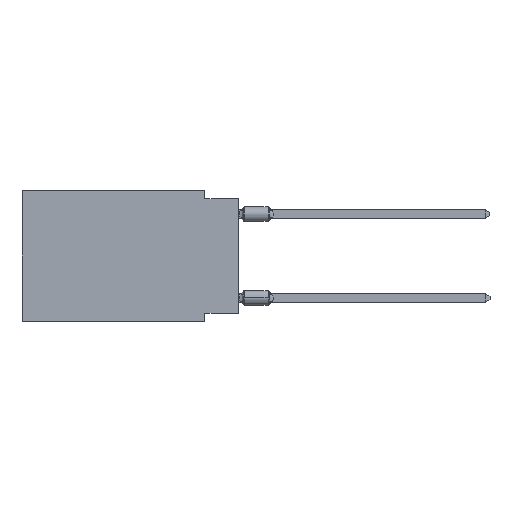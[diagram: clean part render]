
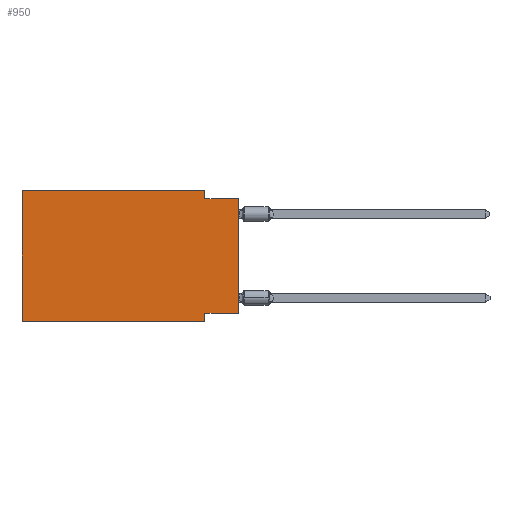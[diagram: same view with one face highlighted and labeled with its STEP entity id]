
A CAD part, left-side view. The second image highlights one B-rep face of the part: STEP entity #950.
In plain terms, the highlighted planar face has unit normal (-1, 0, 0).
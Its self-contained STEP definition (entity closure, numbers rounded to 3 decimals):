
#27 = VERTEX_POINT ( 'NONE', #13532 ) ;
#347 = CARTESIAN_POINT ( 'NONE',  ( 0., 16.383, -9.906 ) ) ;
#525 = EDGE_LOOP ( 'NONE', ( #1098, #870, #3575, #7750, #797, #1047, #6984, #12785 ) ) ;
#543 = DIRECTION ( 'NONE',  ( 0., 0., -1. ) ) ;
#556 = DIRECTION ( 'NONE',  ( 0., 0., -1. ) ) ;
#703 = LINE ( 'NONE', #8393, #5016 ) ;
#797 = ORIENTED_EDGE ( 'NONE', *, *, #9478, .F. ) ;
#870 = ORIENTED_EDGE ( 'NONE', *, *, #2274, .F. ) ;
#950 = ADVANCED_FACE ( 'NONE', ( #11887 ), #1693, .F. ) ;
#1047 = ORIENTED_EDGE ( 'NONE', *, *, #3171, .T. ) ;
#1081 = VERTEX_POINT ( 'NONE', #11957 ) ;
#1098 = ORIENTED_EDGE ( 'NONE', *, *, #9392, .T. ) ;
#1195 = LINE ( 'NONE', #8754, #2964 ) ;
#1472 = DIRECTION ( 'NONE',  ( 0., 0., 1. ) ) ;
#1693 = PLANE ( 'NONE',  #1806 ) ;
#1806 = AXIS2_PLACEMENT_3D ( 'NONE', #8456, #10587, #543 ) ;
#1985 = VECTOR ( 'NONE', #11411, 1000. ) ;
#2074 = DIRECTION ( 'NONE',  ( 0., 1., 0. ) ) ;
#2218 = LINE ( 'NONE', #12042, #13100 ) ;
#2274 = EDGE_CURVE ( 'NONE', #12312, #4316, #8478, .T. ) ;
#2418 = CARTESIAN_POINT ( 'NONE',  ( 0., 16.383, 0. ) ) ;
#2615 = EDGE_CURVE ( 'NONE', #10308, #27, #11003, .T. ) ;
#2964 = VECTOR ( 'NONE', #6641, 1000. ) ;
#3171 = EDGE_CURVE ( 'NONE', #9351, #27, #6946, .T. ) ;
#3351 = DIRECTION ( 'NONE',  ( 0., 0., -1. ) ) ;
#3575 = ORIENTED_EDGE ( 'NONE', *, *, #12640, .F. ) ;
#4316 = VERTEX_POINT ( 'NONE', #9260 ) ;
#4456 = VERTEX_POINT ( 'NONE', #5188 ) ;
#4783 = DIRECTION ( 'NONE',  ( 0., -1., 0. ) ) ;
#5016 = VECTOR ( 'NONE', #556, 1000. ) ;
#5188 = CARTESIAN_POINT ( 'NONE',  ( 0., 0., -9.271 ) ) ;
#5266 = EDGE_CURVE ( 'NONE', #4456, #10308, #2218, .T. ) ;
#5521 = CARTESIAN_POINT ( 'NONE',  ( 0., 16.383, 0. ) ) ;
#5980 = VECTOR ( 'NONE', #1472, 1000. ) ;
#6297 = VECTOR ( 'NONE', #3351, 1000. ) ;
#6641 = DIRECTION ( 'NONE',  ( 0., 0., 1. ) ) ;
#6946 = LINE ( 'NONE', #347, #7699 ) ;
#6984 = ORIENTED_EDGE ( 'NONE', *, *, #2615, .F. ) ;
#7699 = VECTOR ( 'NONE', #4783, 1000. ) ;
#7725 = CARTESIAN_POINT ( 'NONE',  ( 0., 16.383, -9.906 ) ) ;
#7750 = ORIENTED_EDGE ( 'NONE', *, *, #12062, .F. ) ;
#8393 = CARTESIAN_POINT ( 'NONE',  ( 0., 2.54, 0. ) ) ;
#8456 = CARTESIAN_POINT ( 'NONE',  ( 0., 16.383, 0. ) ) ;
#8478 = LINE ( 'NONE', #10958, #8606 ) ;
#8524 = VERTEX_POINT ( 'NONE', #5521 ) ;
#8606 = VECTOR ( 'NONE', #12048, 1000. ) ;
#8754 = CARTESIAN_POINT ( 'NONE',  ( 0., 0., 0. ) ) ;
#9260 = CARTESIAN_POINT ( 'NONE',  ( 0., 0., -0.635 ) ) ;
#9344 = CARTESIAN_POINT ( 'NONE',  ( 0., 2.54, -9.271 ) ) ;
#9351 = VERTEX_POINT ( 'NONE', #7725 ) ;
#9392 = EDGE_CURVE ( 'NONE', #4456, #4316, #1195, .T. ) ;
#9478 = EDGE_CURVE ( 'NONE', #9351, #8524, #11302, .T. ) ;
#9874 = CARTESIAN_POINT ( 'NONE',  ( 0., 2.54, -0.635 ) ) ;
#10308 = VERTEX_POINT ( 'NONE', #9344 ) ;
#10587 = DIRECTION ( 'NONE',  ( 1., 0., 0. ) ) ;
#10958 = CARTESIAN_POINT ( 'NONE',  ( 0., 0., -0.635 ) ) ;
#11003 = LINE ( 'NONE', #13313, #6297 ) ;
#11273 = CARTESIAN_POINT ( 'NONE',  ( 0., 16.383, 0. ) ) ;
#11302 = LINE ( 'NONE', #2418, #5980 ) ;
#11411 = DIRECTION ( 'NONE',  ( 0., -1., 0. ) ) ;
#11887 = FACE_OUTER_BOUND ( 'NONE', #525, .T. ) ;
#11957 = CARTESIAN_POINT ( 'NONE',  ( 0., 2.54, 0. ) ) ;
#12042 = CARTESIAN_POINT ( 'NONE',  ( 0., 0., -9.271 ) ) ;
#12048 = DIRECTION ( 'NONE',  ( 0., -1., 0. ) ) ;
#12062 = EDGE_CURVE ( 'NONE', #8524, #1081, #13512, .T. ) ;
#12312 = VERTEX_POINT ( 'NONE', #9874 ) ;
#12640 = EDGE_CURVE ( 'NONE', #1081, #12312, #703, .T. ) ;
#12785 = ORIENTED_EDGE ( 'NONE', *, *, #5266, .F. ) ;
#13100 = VECTOR ( 'NONE', #2074, 1000. ) ;
#13313 = CARTESIAN_POINT ( 'NONE',  ( 0., 2.54, -9.906 ) ) ;
#13512 = LINE ( 'NONE', #11273, #1985 ) ;
#13532 = CARTESIAN_POINT ( 'NONE',  ( 0., 2.54, -9.906 ) ) ;
